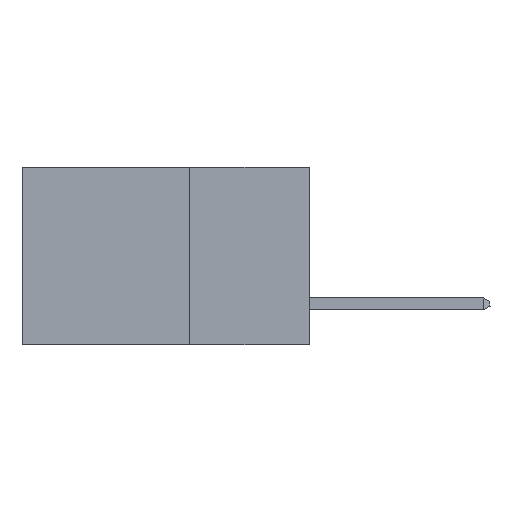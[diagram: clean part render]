
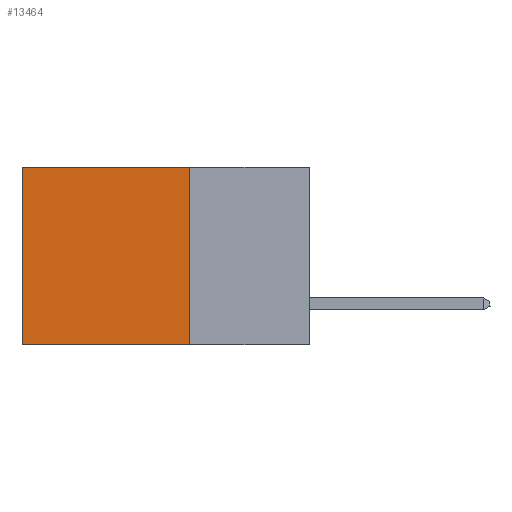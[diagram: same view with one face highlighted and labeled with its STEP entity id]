
A CAD part, left-side view. The second image highlights one B-rep face of the part: STEP entity #13464.
In plain terms, the highlighted planar face has unit normal (-1, 0, 0).
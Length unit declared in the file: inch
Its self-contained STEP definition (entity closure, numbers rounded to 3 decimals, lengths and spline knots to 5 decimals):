
#239 = ORIENTED_EDGE ( 'NONE', *, *, #2501, .F. ) ;
#324 = CARTESIAN_POINT ( 'NONE',  ( 0.2875, 0.25, -0.37 ) ) ;
#360 = CARTESIAN_POINT ( 'NONE',  ( 0.2875, 0.25, 0. ) ) ;
#581 = PLANE ( 'NONE',  #6628 ) ;
#2481 = VECTOR ( 'NONE', #5334, 39.37008 ) ;
#2501 = EDGE_CURVE ( 'NONE', #13796, #6795, #7988, .T. ) ;
#2558 = VECTOR ( 'NONE', #6027, 39.37008 ) ;
#2909 = VECTOR ( 'NONE', #15108, 39.37008 ) ;
#3194 = EDGE_CURVE ( 'NONE', #3912, #6795, #13429, .T. ) ;
#3201 = ORIENTED_EDGE ( 'NONE', *, *, #13050, .F. ) ;
#3912 = VERTEX_POINT ( 'NONE', #8984 ) ;
#4384 = CARTESIAN_POINT ( 'NONE',  ( 0.2875, 0.25, 0. ) ) ;
#5334 = DIRECTION ( 'NONE',  ( 0., 1., 0. ) ) ;
#5449 = CARTESIAN_POINT ( 'NONE',  ( 0.2875, 0.6, -0.37 ) ) ;
#5785 = ORIENTED_EDGE ( 'NONE', *, *, #8878, .T. ) ;
#6027 = DIRECTION ( 'NONE',  ( 0., 0., -1. ) ) ;
#6628 = AXIS2_PLACEMENT_3D ( 'NONE', #11587, #7788, #12781 ) ;
#6647 = CARTESIAN_POINT ( 'NONE',  ( 0.2875, 0.25, 0. ) ) ;
#6795 = VERTEX_POINT ( 'NONE', #5449 ) ;
#7491 = VERTEX_POINT ( 'NONE', #4384 ) ;
#7532 = CARTESIAN_POINT ( 'NONE',  ( 0.2875, 0.25, -0.37 ) ) ;
#7788 = DIRECTION ( 'NONE',  ( 1., 0., 0. ) ) ;
#7988 = LINE ( 'NONE', #324, #10837 ) ;
#8084 = LINE ( 'NONE', #6647, #2481 ) ;
#8696 = DIRECTION ( 'NONE',  ( 0., 1., 0. ) ) ;
#8878 = EDGE_CURVE ( 'NONE', #7491, #3912, #8084, .T. ) ;
#8984 = CARTESIAN_POINT ( 'NONE',  ( 0.2875, 0.6, 0. ) ) ;
#10837 = VECTOR ( 'NONE', #8696, 39.37008 ) ;
#11587 = CARTESIAN_POINT ( 'NONE',  ( 0.2875, 0.25, 0. ) ) ;
#11890 = CARTESIAN_POINT ( 'NONE',  ( 0.2875, 0.6, 0. ) ) ;
#12781 = DIRECTION ( 'NONE',  ( 0., 0., -1. ) ) ;
#13050 = EDGE_CURVE ( 'NONE', #7491, #13796, #13620, .T. ) ;
#13429 = LINE ( 'NONE', #11890, #2558 ) ;
#13464 = ADVANCED_FACE ( 'NONE', ( #14263 ), #581, .F. ) ;
#13499 = EDGE_LOOP ( 'NONE', ( #14647, #239, #3201, #5785 ) ) ;
#13620 = LINE ( 'NONE', #360, #2909 ) ;
#13796 = VERTEX_POINT ( 'NONE', #7532 ) ;
#14263 = FACE_OUTER_BOUND ( 'NONE', #13499, .T. ) ;
#14647 = ORIENTED_EDGE ( 'NONE', *, *, #3194, .T. ) ;
#15108 = DIRECTION ( 'NONE',  ( 0., 0., -1. ) ) ;
